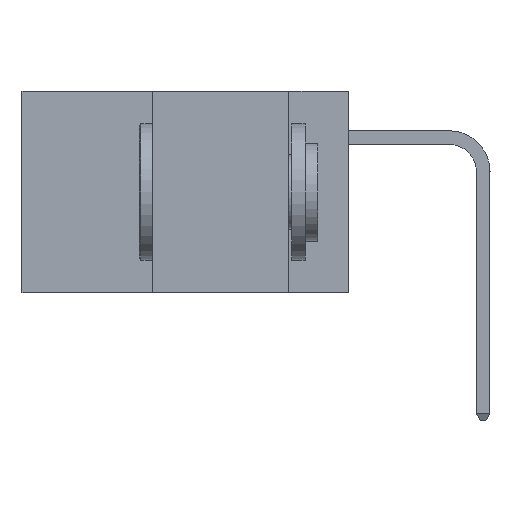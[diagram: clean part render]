
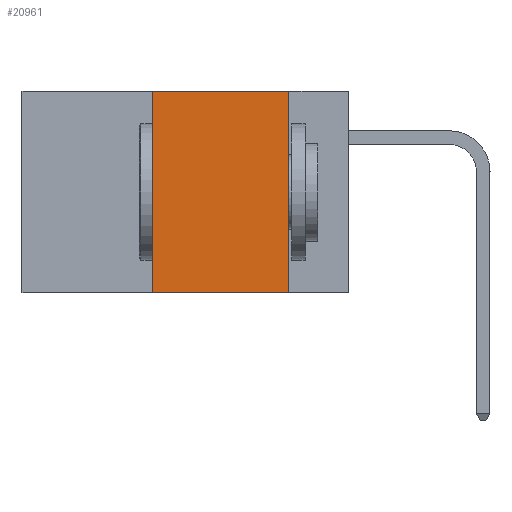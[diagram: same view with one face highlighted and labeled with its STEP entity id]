
A CAD part, left-side view. The second image highlights one B-rep face of the part: STEP entity #20961.
In plain terms, the highlighted planar face has unit normal (-1, 0, 0).
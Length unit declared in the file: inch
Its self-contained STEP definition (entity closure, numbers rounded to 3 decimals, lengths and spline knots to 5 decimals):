
#1244 = CARTESIAN_POINT ( 'NONE',  ( 0., 0.11, -0.37 ) ) ;
#1815 = LINE ( 'NONE', #35211, #18051 ) ;
#1869 = DIRECTION ( 'NONE',  ( 0., 0., -1. ) ) ;
#2193 = CARTESIAN_POINT ( 'NONE',  ( 0., 0.36, 0. ) ) ;
#2230 = DIRECTION ( 'NONE',  ( 0., -1., 0. ) ) ;
#5354 = AXIS2_PLACEMENT_3D ( 'NONE', #38923, #24020, #1869 ) ;
#8420 = CARTESIAN_POINT ( 'NONE',  ( 0., 0.6, -0.37 ) ) ;
#10293 = VERTEX_POINT ( 'NONE', #30097 ) ;
#11743 = LINE ( 'NONE', #11791, #43493 ) ;
#11791 = CARTESIAN_POINT ( 'NONE',  ( 0., 0.11, 0. ) ) ;
#12179 = DIRECTION ( 'NONE',  ( 0., -1., 0. ) ) ;
#14107 = ORIENTED_EDGE ( 'NONE', *, *, #41392, .T. ) ;
#15757 = EDGE_LOOP ( 'NONE', ( #34853, #34718, #18663, #14107 ) ) ;
#16278 = VERTEX_POINT ( 'NONE', #18781 ) ;
#17260 = VERTEX_POINT ( 'NONE', #2193 ) ;
#18051 = VECTOR ( 'NONE', #2230, 39.37008 ) ;
#18663 = ORIENTED_EDGE ( 'NONE', *, *, #38644, .F. ) ;
#18717 = DIRECTION ( 'NONE',  ( 0., 0., -1. ) ) ;
#18781 = CARTESIAN_POINT ( 'NONE',  ( 0., 0.11, 0. ) ) ;
#20961 = ADVANCED_FACE ( 'NONE', ( #28804 ), #46133, .F. ) ;
#23816 = DIRECTION ( 'NONE',  ( 0., 0., 1. ) ) ;
#24020 = DIRECTION ( 'NONE',  ( 1., 0., 0. ) ) ;
#25471 = LINE ( 'NONE', #27708, #34135 ) ;
#27708 = CARTESIAN_POINT ( 'NONE',  ( 0., 0.36, 0. ) ) ;
#28804 = FACE_OUTER_BOUND ( 'NONE', #15757, .T. ) ;
#30097 = CARTESIAN_POINT ( 'NONE',  ( 0., 0.36, -0.37 ) ) ;
#32102 = EDGE_CURVE ( 'NONE', #16278, #44985, #11743, .T. ) ;
#34135 = VECTOR ( 'NONE', #23816, 39.37008 ) ;
#34718 = ORIENTED_EDGE ( 'NONE', *, *, #45939, .F. ) ;
#34853 = ORIENTED_EDGE ( 'NONE', *, *, #32102, .F. ) ;
#35211 = CARTESIAN_POINT ( 'NONE',  ( 0., 0.6, 0. ) ) ;
#38644 = EDGE_CURVE ( 'NONE', #10293, #17260, #25471, .T. ) ;
#38923 = CARTESIAN_POINT ( 'NONE',  ( 0., 0.6, 0. ) ) ;
#40243 = LINE ( 'NONE', #8420, #41931 ) ;
#41392 = EDGE_CURVE ( 'NONE', #10293, #44985, #40243, .T. ) ;
#41931 = VECTOR ( 'NONE', #12179, 39.37008 ) ;
#43493 = VECTOR ( 'NONE', #18717, 39.37008 ) ;
#44985 = VERTEX_POINT ( 'NONE', #1244 ) ;
#45939 = EDGE_CURVE ( 'NONE', #17260, #16278, #1815, .T. ) ;
#46133 = PLANE ( 'NONE',  #5354 ) ;
